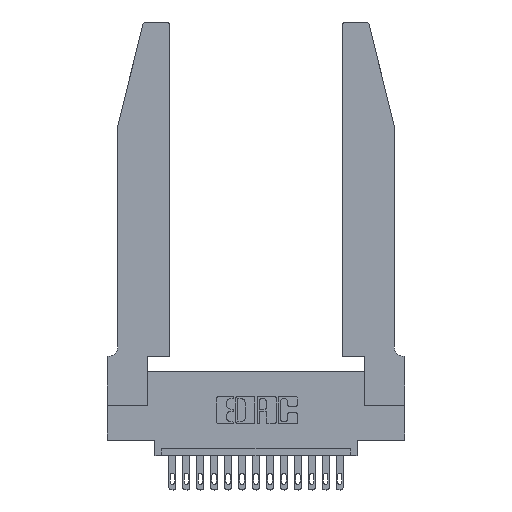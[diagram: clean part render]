
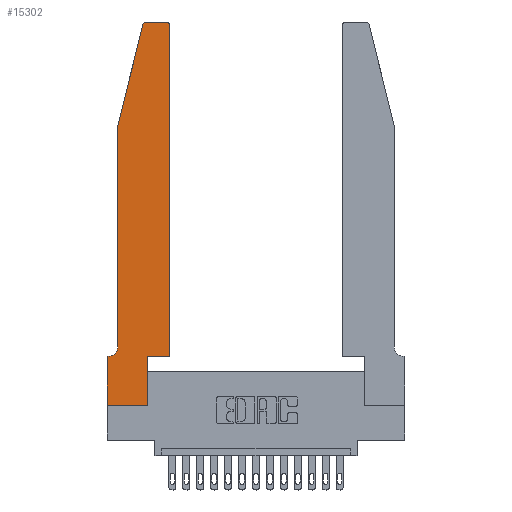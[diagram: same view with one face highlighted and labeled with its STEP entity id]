
A CAD part, top view. The second image highlights one B-rep face of the part: STEP entity #15302.
In plain terms, the highlighted planar face has unit normal (0, 0, 1).
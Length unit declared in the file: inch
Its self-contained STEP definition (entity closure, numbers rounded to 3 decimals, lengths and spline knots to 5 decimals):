
#422 = AXIS2_PLACEMENT_3D ( 'NONE', #11139, #7053, #8343 ) ;
#491 = DIRECTION ( 'NONE',  ( 1., 0., 0. ) ) ;
#625 = CIRCLE ( 'NONE', #4222, 0.07 ) ;
#732 = ORIENTED_EDGE ( 'NONE', *, *, #10437, .T. ) ;
#773 = VERTEX_POINT ( 'NONE', #12353 ) ;
#777 = VECTOR ( 'NONE', #8393, 39.37008 ) ;
#969 = CARTESIAN_POINT ( 'NONE',  ( 0.284, 2.75, 0.37 ) ) ;
#1906 = CARTESIAN_POINT ( 'NONE',  ( 0.4505, 0.35, 0.37 ) ) ;
#2124 = CARTESIAN_POINT ( 'NONE',  ( 0.4505, 0.35, 0.37 ) ) ;
#2377 = EDGE_CURVE ( 'NONE', #773, #3683, #625, .T. ) ;
#2389 = VECTOR ( 'NONE', #16710, 39.37008 ) ;
#2497 = ORIENTED_EDGE ( 'NONE', *, *, #12286, .T. ) ;
#2535 = ORIENTED_EDGE ( 'NONE', *, *, #11818, .T. ) ;
#2692 = CARTESIAN_POINT ( 'NONE',  ( 0., 0., 0.37 ) ) ;
#3007 = ORIENTED_EDGE ( 'NONE', *, *, #11363, .T. ) ;
#3176 = CARTESIAN_POINT ( 'NONE',  ( 0.2865, 0.35, 0.37 ) ) ;
#3273 = VECTOR ( 'NONE', #17744, 39.37008 ) ;
#3281 = CARTESIAN_POINT ( 'NONE',  ( 0.4205, 2.72, 0.37 ) ) ;
#3299 = CARTESIAN_POINT ( 'NONE',  ( 0.0755, 0.35, 0.37 ) ) ;
#3336 = CIRCLE ( 'NONE', #12654, 0.03 ) ;
#3465 = LINE ( 'NONE', #5884, #8571 ) ;
#3527 = DIRECTION ( 'NONE',  ( 0., 0., 1. ) ) ;
#3546 = CARTESIAN_POINT ( 'NONE',  ( 0.0755, 2., 0.37 ) ) ;
#3608 = VECTOR ( 'NONE', #5311, 39.37008 ) ;
#3680 = CARTESIAN_POINT ( 'NONE',  ( 0.0755, 2., 0.37 ) ) ;
#3683 = VERTEX_POINT ( 'NONE', #10465 ) ;
#3727 = LINE ( 'NONE', #3680, #5509 ) ;
#3780 = EDGE_CURVE ( 'NONE', #14427, #13124, #6814, .T. ) ;
#4222 = AXIS2_PLACEMENT_3D ( 'NONE', #13627, #5073, #17965 ) ;
#4371 = CARTESIAN_POINT ( 'NONE',  ( 0., 0., 0.37 ) ) ;
#4572 = ORIENTED_EDGE ( 'NONE', *, *, #3780, .T. ) ;
#4824 = VERTEX_POINT ( 'NONE', #17555 ) ;
#5073 = DIRECTION ( 'NONE',  ( 0., 0., -1. ) ) ;
#5222 = EDGE_CURVE ( 'NONE', #3683, #13176, #5522, .T. ) ;
#5311 = DIRECTION ( 'NONE',  ( 0., -1., 0. ) ) ;
#5509 = VECTOR ( 'NONE', #15092, 39.37008 ) ;
#5522 = LINE ( 'NONE', #3299, #3273 ) ;
#5884 = CARTESIAN_POINT ( 'NONE',  ( 0.2865, 0.35, 0.37 ) ) ;
#6073 = VERTEX_POINT ( 'NONE', #12689 ) ;
#6256 = DIRECTION ( 'NONE',  ( 1., 0., 0. ) ) ;
#6338 = CARTESIAN_POINT ( 'NONE',  ( 0., 0., 0.37 ) ) ;
#6370 = DIRECTION ( 'NONE',  ( 0., 1., 0. ) ) ;
#6545 = FACE_OUTER_BOUND ( 'NONE', #11873, .T. ) ;
#6705 = EDGE_CURVE ( 'NONE', #18386, #14427, #13445, .T. ) ;
#6741 = EDGE_CURVE ( 'NONE', #15886, #18386, #9633, .T. ) ;
#6807 = CARTESIAN_POINT ( 'NONE',  ( 0.4505, 0.35, 0.37 ) ) ;
#6814 = CIRCLE ( 'NONE', #11017, 0.03 ) ;
#6824 = ORIENTED_EDGE ( 'NONE', *, *, #2377, .T. ) ;
#7053 = DIRECTION ( 'NONE',  ( 0., 0., 1. ) ) ;
#7225 = EDGE_CURVE ( 'NONE', #13176, #18524, #17464, .T. ) ;
#7653 = DIRECTION ( 'NONE',  ( 0., 0., 1. ) ) ;
#7708 = ORIENTED_EDGE ( 'NONE', *, *, #6741, .T. ) ;
#7812 = CARTESIAN_POINT ( 'NONE',  ( 0.4505, 2.72, 0.37 ) ) ;
#7835 = VERTEX_POINT ( 'NONE', #17689 ) ;
#7985 = CARTESIAN_POINT ( 'NONE',  ( 0.2605, 2.75, 0.37 ) ) ;
#8343 = DIRECTION ( 'NONE',  ( 1., 0., 0. ) ) ;
#8393 = DIRECTION ( 'NONE',  ( 0., -1., 0. ) ) ;
#8571 = VECTOR ( 'NONE', #8604, 39.37008 ) ;
#8604 = DIRECTION ( 'NONE',  ( 0., 1., 0. ) ) ;
#8869 = EDGE_CURVE ( 'NONE', #14655, #7835, #3336, .T. ) ;
#8906 = CARTESIAN_POINT ( 'NONE',  ( 0.4205, 2.75, 0.37 ) ) ;
#8953 = VECTOR ( 'NONE', #6370, 39.37008 ) ;
#9546 = VECTOR ( 'NONE', #16632, 39.37008 ) ;
#9633 = LINE ( 'NONE', #6807, #10282 ) ;
#9813 = EDGE_CURVE ( 'NONE', #18524, #6073, #13358, .T. ) ;
#9995 = ORIENTED_EDGE ( 'NONE', *, *, #6705, .T. ) ;
#10245 = ORIENTED_EDGE ( 'NONE', *, *, #5222, .T. ) ;
#10282 = VECTOR ( 'NONE', #18252, 39.37008 ) ;
#10437 = EDGE_CURVE ( 'NONE', #13124, #14655, #16932, .T. ) ;
#10465 = CARTESIAN_POINT ( 'NONE',  ( 0.0055, 0.35, 0.37 ) ) ;
#11005 = CARTESIAN_POINT ( 'NONE',  ( 0., 0.35, 0.37 ) ) ;
#11017 = AXIS2_PLACEMENT_3D ( 'NONE', #3281, #3527, #6256 ) ;
#11139 = CARTESIAN_POINT ( 'NONE',  ( 0., 0.35, 0.37 ) ) ;
#11363 = EDGE_CURVE ( 'NONE', #6073, #15886, #3465, .T. ) ;
#11818 = EDGE_CURVE ( 'NONE', #4824, #773, #15989, .T. ) ;
#11873 = EDGE_LOOP ( 'NONE', ( #732, #12044, #2497, #2535, #6824, #10245, #15461, #16758, #3007, #7708, #9995, #4572 ) ) ;
#12044 = ORIENTED_EDGE ( 'NONE', *, *, #8869, .T. ) ;
#12286 = EDGE_CURVE ( 'NONE', #7835, #4824, #3727, .T. ) ;
#12353 = CARTESIAN_POINT ( 'NONE',  ( 0.0755, 0.42, 0.37 ) ) ;
#12654 = AXIS2_PLACEMENT_3D ( 'NONE', #17737, #7653, #491 ) ;
#12689 = CARTESIAN_POINT ( 'NONE',  ( 0.2865, 0., 0.37 ) ) ;
#13124 = VERTEX_POINT ( 'NONE', #8906 ) ;
#13176 = VERTEX_POINT ( 'NONE', #11005 ) ;
#13358 = LINE ( 'NONE', #4371, #9546 ) ;
#13445 = LINE ( 'NONE', #2124, #8953 ) ;
#13627 = CARTESIAN_POINT ( 'NONE',  ( 0.0055, 0.42, 0.37 ) ) ;
#14110 = PLANE ( 'NONE',  #422 ) ;
#14427 = VERTEX_POINT ( 'NONE', #7812 ) ;
#14655 = VERTEX_POINT ( 'NONE', #969 ) ;
#15092 = DIRECTION ( 'NONE',  ( -0.239, -0.971, 0. ) ) ;
#15302 = ADVANCED_FACE ( 'NONE', ( #6545 ), #14110, .T. ) ;
#15461 = ORIENTED_EDGE ( 'NONE', *, *, #7225, .T. ) ;
#15886 = VERTEX_POINT ( 'NONE', #3176 ) ;
#15989 = LINE ( 'NONE', #3546, #777 ) ;
#16632 = DIRECTION ( 'NONE',  ( 1., 0., 0. ) ) ;
#16710 = DIRECTION ( 'NONE',  ( -1., 0., 0. ) ) ;
#16758 = ORIENTED_EDGE ( 'NONE', *, *, #9813, .T. ) ;
#16932 = LINE ( 'NONE', #7985, #2389 ) ;
#17464 = LINE ( 'NONE', #2692, #3608 ) ;
#17555 = CARTESIAN_POINT ( 'NONE',  ( 0.0755, 2., 0.37 ) ) ;
#17689 = CARTESIAN_POINT ( 'NONE',  ( 0.25487, 2.72718, 0.37 ) ) ;
#17737 = CARTESIAN_POINT ( 'NONE',  ( 0.284, 2.72, 0.37 ) ) ;
#17744 = DIRECTION ( 'NONE',  ( -1., 0., 0. ) ) ;
#17965 = DIRECTION ( 'NONE',  ( -1., 0., 0. ) ) ;
#18252 = DIRECTION ( 'NONE',  ( 1., 0., 0. ) ) ;
#18386 = VERTEX_POINT ( 'NONE', #1906 ) ;
#18524 = VERTEX_POINT ( 'NONE', #6338 ) ;
